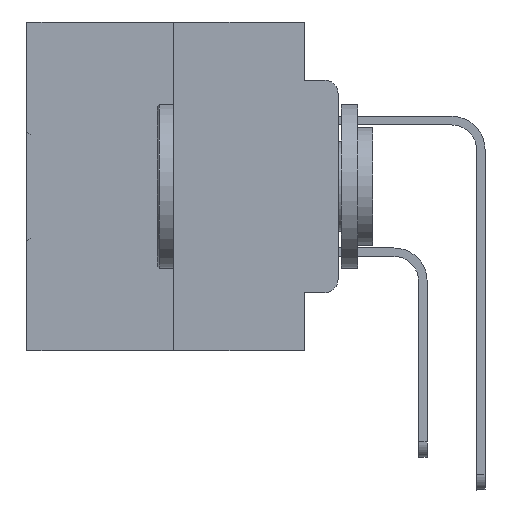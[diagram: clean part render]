
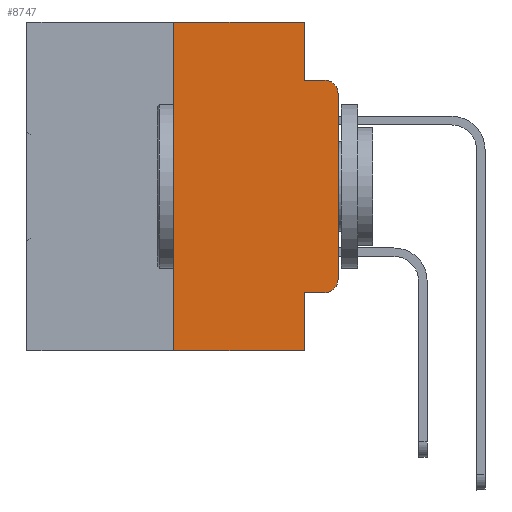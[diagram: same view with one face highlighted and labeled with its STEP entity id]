
A CAD part, left-side view. The second image highlights one B-rep face of the part: STEP entity #8747.
In plain terms, the highlighted planar face has unit normal (-1, 0, 0).
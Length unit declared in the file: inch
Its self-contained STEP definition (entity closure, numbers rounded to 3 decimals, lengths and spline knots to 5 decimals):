
#143 = ORIENTED_EDGE ( 'NONE', *, *, #14201, .F. ) ;
#185 = CARTESIAN_POINT ( 'NONE',  ( 0., 0.051, -0.0885 ) ) ;
#852 = LINE ( 'NONE', #20046, #6935 ) ;
#992 = CARTESIAN_POINT ( 'NONE',  ( 0., 0.02, -0.0885 ) ) ;
#1660 = AXIS2_PLACEMENT_3D ( 'NONE', #33036, #17666, #2306 ) ;
#1899 = VECTOR ( 'NONE', #16015, 39.37008 ) ;
#2081 = DIRECTION ( 'NONE',  ( 0., 0., -1. ) ) ;
#2212 = ORIENTED_EDGE ( 'NONE', *, *, #19872, .T. ) ;
#2306 = DIRECTION ( 'NONE',  ( 0., 0., -1. ) ) ;
#2723 = VERTEX_POINT ( 'NONE', #29307 ) ;
#3016 = VECTOR ( 'NONE', #6581, 39.37008 ) ;
#3549 = VERTEX_POINT ( 'NONE', #4535 ) ;
#4535 = CARTESIAN_POINT ( 'NONE',  ( 0., 0.051, 0. ) ) ;
#4580 = CARTESIAN_POINT ( 'NONE',  ( 0., 0., 0. ) ) ;
#4636 = VECTOR ( 'NONE', #5471, 39.37008 ) ;
#4686 = CIRCLE ( 'NONE', #10250, 0.02 ) ;
#5471 = DIRECTION ( 'NONE',  ( 0., -1., 0. ) ) ;
#5487 = ORIENTED_EDGE ( 'NONE', *, *, #32321, .F. ) ;
#6342 = CARTESIAN_POINT ( 'NONE',  ( 0., 0.25, -0.5 ) ) ;
#6360 = VECTOR ( 'NONE', #7240, 39.37008 ) ;
#6581 = DIRECTION ( 'NONE',  ( 0., 0., -1. ) ) ;
#6859 = EDGE_LOOP ( 'NONE', ( #28789, #2212, #25111, #5487, #143, #13806, #29199, #16252, #10996, #14220 ) ) ;
#6891 = VECTOR ( 'NONE', #9501, 39.37008 ) ;
#6935 = VECTOR ( 'NONE', #2081, 39.37008 ) ;
#6992 = CARTESIAN_POINT ( 'NONE',  ( 0., 0.473, 0. ) ) ;
#7240 = DIRECTION ( 'NONE',  ( 0., 0., 1. ) ) ;
#7254 = DIRECTION ( 'NONE',  ( 0., -1., 0. ) ) ;
#7340 = CARTESIAN_POINT ( 'NONE',  ( 0., 0.051, -0.4115 ) ) ;
#7456 = EDGE_CURVE ( 'NONE', #18464, #15345, #18262, .T. ) ;
#7854 = DIRECTION ( 'NONE',  ( -1., 0., 0. ) ) ;
#8481 = VERTEX_POINT ( 'NONE', #24990 ) ;
#8747 = ADVANCED_FACE ( 'NONE', ( #31074 ), #31205, .F. ) ;
#9109 = EDGE_CURVE ( 'NONE', #28890, #2723, #26630, .T. ) ;
#9501 = DIRECTION ( 'NONE',  ( 0., -1., 0. ) ) ;
#10011 = CARTESIAN_POINT ( 'NONE',  ( 0., 0.02, -0.4115 ) ) ;
#10065 = VECTOR ( 'NONE', #7254, 39.37008 ) ;
#10250 = AXIS2_PLACEMENT_3D ( 'NONE', #23201, #7854, #25807 ) ;
#10567 = LINE ( 'NONE', #32259, #3016 ) ;
#10771 = DIRECTION ( 'NONE',  ( 0., 0., -1. ) ) ;
#10996 = ORIENTED_EDGE ( 'NONE', *, *, #25737, .T. ) ;
#12214 = DIRECTION ( 'NONE',  ( 0., 0., 1. ) ) ;
#12991 = VECTOR ( 'NONE', #12214, 39.37008 ) ;
#13397 = CARTESIAN_POINT ( 'NONE',  ( 0., 0.051, -0.4115 ) ) ;
#13635 = EDGE_CURVE ( 'NONE', #28890, #18576, #16934, .T. ) ;
#13806 = ORIENTED_EDGE ( 'NONE', *, *, #9109, .F. ) ;
#14201 = EDGE_CURVE ( 'NONE', #2723, #3549, #20548, .T. ) ;
#14220 = ORIENTED_EDGE ( 'NONE', *, *, #30485, .T. ) ;
#15157 = AXIS2_PLACEMENT_3D ( 'NONE', #21066, #26235, #10771 ) ;
#15345 = VERTEX_POINT ( 'NONE', #992 ) ;
#16015 = DIRECTION ( 'NONE',  ( 0., -1., 0. ) ) ;
#16252 = ORIENTED_EDGE ( 'NONE', *, *, #20776, .F. ) ;
#16934 = LINE ( 'NONE', #27851, #10065 ) ;
#17666 = DIRECTION ( 'NONE',  ( -1., 0., 0. ) ) ;
#18262 = LINE ( 'NONE', #185, #4636 ) ;
#18393 = EDGE_CURVE ( 'NONE', #28291, #8481, #20718, .T. ) ;
#18464 = VERTEX_POINT ( 'NONE', #22816 ) ;
#18576 = VERTEX_POINT ( 'NONE', #23286 ) ;
#19872 = EDGE_CURVE ( 'NONE', #8481, #15345, #4686, .T. ) ;
#20017 = CARTESIAN_POINT ( 'NONE',  ( 0., 0.25, 0. ) ) ;
#20046 = CARTESIAN_POINT ( 'NONE',  ( 0., 0.051, 0. ) ) ;
#20548 = LINE ( 'NONE', #6992, #6891 ) ;
#20718 = LINE ( 'NONE', #4580, #12991 ) ;
#20776 = EDGE_CURVE ( 'NONE', #31113, #18576, #10567, .T. ) ;
#21066 = CARTESIAN_POINT ( 'NONE',  ( 0., 0.473, 0. ) ) ;
#21265 = CARTESIAN_POINT ( 'NONE',  ( 0., 0., -0.3915 ) ) ;
#21596 = LINE ( 'NONE', #13397, #1899 ) ;
#22816 = CARTESIAN_POINT ( 'NONE',  ( 0., 0.051, -0.0885 ) ) ;
#23201 = CARTESIAN_POINT ( 'NONE',  ( 0., 0.02, -0.1085 ) ) ;
#23286 = CARTESIAN_POINT ( 'NONE',  ( 0., 0.051, -0.5 ) ) ;
#24221 = VERTEX_POINT ( 'NONE', #10011 ) ;
#24990 = CARTESIAN_POINT ( 'NONE',  ( 0., 0., -0.1085 ) ) ;
#25111 = ORIENTED_EDGE ( 'NONE', *, *, #7456, .F. ) ;
#25737 = EDGE_CURVE ( 'NONE', #31113, #24221, #21596, .T. ) ;
#25807 = DIRECTION ( 'NONE',  ( 0., 0., -1. ) ) ;
#26235 = DIRECTION ( 'NONE',  ( 1., 0., 0. ) ) ;
#26630 = LINE ( 'NONE', #20017, #6360 ) ;
#27770 = CIRCLE ( 'NONE', #1660, 0.02 ) ;
#27851 = CARTESIAN_POINT ( 'NONE',  ( 0., 0.473, -0.5 ) ) ;
#28291 = VERTEX_POINT ( 'NONE', #21265 ) ;
#28789 = ORIENTED_EDGE ( 'NONE', *, *, #18393, .T. ) ;
#28890 = VERTEX_POINT ( 'NONE', #6342 ) ;
#29199 = ORIENTED_EDGE ( 'NONE', *, *, #13635, .T. ) ;
#29307 = CARTESIAN_POINT ( 'NONE',  ( 0., 0.25, 0. ) ) ;
#30485 = EDGE_CURVE ( 'NONE', #24221, #28291, #27770, .T. ) ;
#31074 = FACE_OUTER_BOUND ( 'NONE', #6859, .T. ) ;
#31113 = VERTEX_POINT ( 'NONE', #7340 ) ;
#31205 = PLANE ( 'NONE',  #15157 ) ;
#32259 = CARTESIAN_POINT ( 'NONE',  ( 0., 0.051, 0. ) ) ;
#32321 = EDGE_CURVE ( 'NONE', #3549, #18464, #852, .T. ) ;
#33036 = CARTESIAN_POINT ( 'NONE',  ( 0., 0.02, -0.3915 ) ) ;
